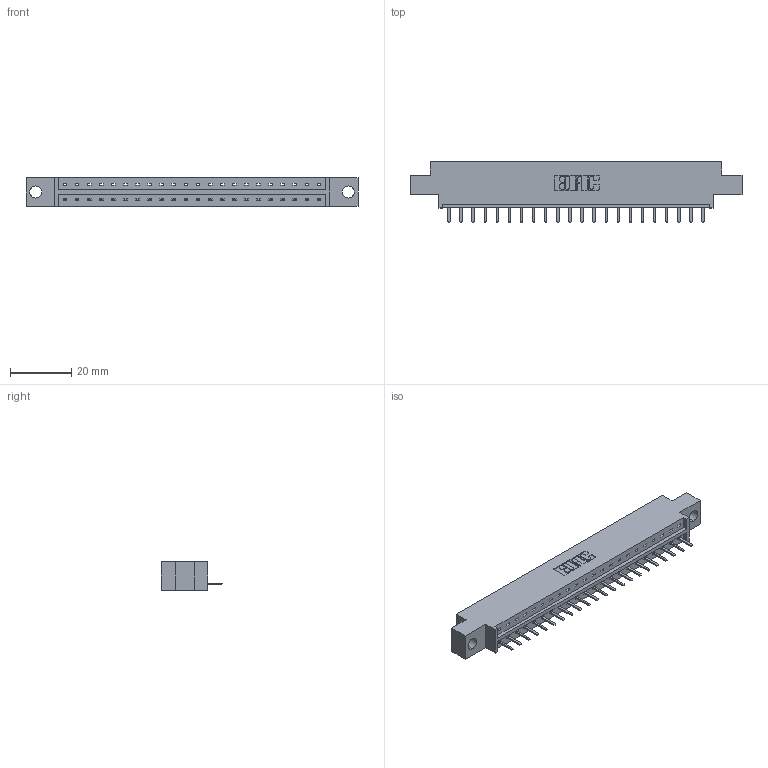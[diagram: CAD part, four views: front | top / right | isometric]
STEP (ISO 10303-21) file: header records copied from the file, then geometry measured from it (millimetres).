
FILE_DESCRIPTION (( 'STEP AP203' ), '1' );
FILE_NAME ('833-022-520-604.STEP', '2020-06-01T16:01:33', ( '' ), ( '' ), 'SwSTEP 2.0', 'SolidWorks 2020', '' );
FILE_SCHEMA (( 'CONFIG_CONTROL_DESIGN' ));
Length unit declared in the file: inch
Products named in the file (3): 833 Part_Offset - .156 Dia - TH; 345-292-001_345-293-120; 833-022-520-604
Assembly tree (23 placements, depth 2):
  833-022-520-604
    833 Part_Offset - .156 Dia - TH
    345-292-001_345-293-120  x22
Bounding box: 108.71 x 20.02 x 9.4 mm (x, y, z)
Volume: 10388.6 mm3; surface area: 10880.7 mm2
Topology: 23 solids, 23 shells, 1482 faces, 4371 edges, 2854 vertices
Faces by surface type: plane 1042, cylinder 440
Entity records: 16285 total; most frequent: CARTESIAN_POINT 2832, ORIENTED_EDGE 2778, DIRECTION 2417, EDGE_CURVE 1389, LINE 1257, VECTOR 1257, VERTEX_POINT 922, AXIS2_PLACEMENT_3D 580
